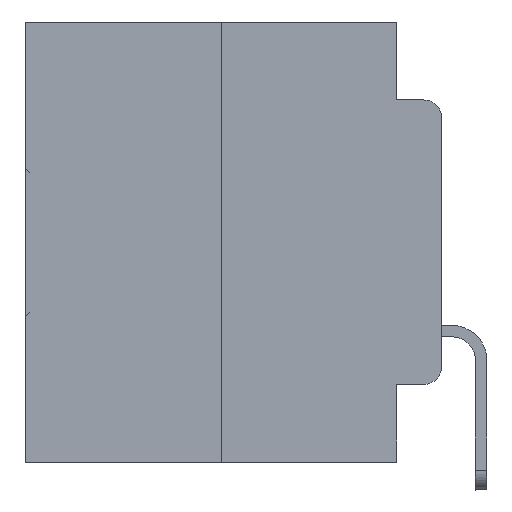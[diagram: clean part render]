
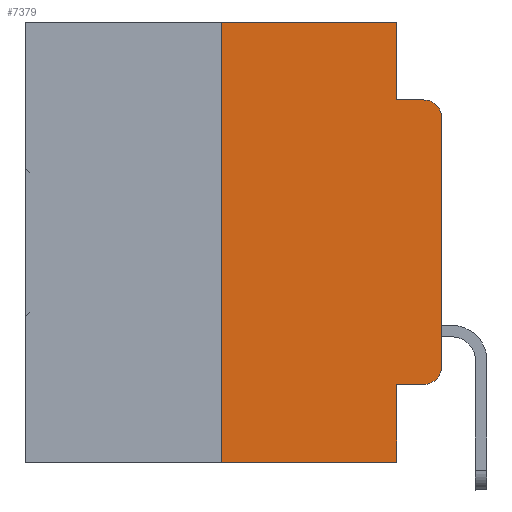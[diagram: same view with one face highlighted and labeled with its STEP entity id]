
A CAD part, left-side view. The second image highlights one B-rep face of the part: STEP entity #7379.
In plain terms, the highlighted planar face has unit normal (-1, 0, 0).
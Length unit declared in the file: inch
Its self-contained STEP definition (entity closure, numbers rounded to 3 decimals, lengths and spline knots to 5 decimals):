
#583 = ORIENTED_EDGE ( 'NONE', *, *, #6155, .T. ) ;
#1033 = DIRECTION ( 'NONE',  ( 0., 0., -1. ) ) ;
#2164 = VERTEX_POINT ( 'NONE', #14094 ) ;
#2459 = CARTESIAN_POINT ( 'NONE',  ( 0., 0.051, -0.4115 ) ) ;
#3384 = CARTESIAN_POINT ( 'NONE',  ( 0., 0.051, 0. ) ) ;
#4004 = ORIENTED_EDGE ( 'NONE', *, *, #21494, .F. ) ;
#4017 = CARTESIAN_POINT ( 'NONE',  ( 0., 0., -0.3915 ) ) ;
#4564 = VERTEX_POINT ( 'NONE', #2459 ) ;
#4943 = VECTOR ( 'NONE', #14178, 39.37008 ) ;
#5143 = LINE ( 'NONE', #29295, #17501 ) ;
#5818 = CARTESIAN_POINT ( 'NONE',  ( 0., 0.02, -0.4115 ) ) ;
#6155 = EDGE_CURVE ( 'NONE', #23217, #22985, #13367, .T. ) ;
#6268 = DIRECTION ( 'NONE',  ( -1., 0., 0. ) ) ;
#6496 = VECTOR ( 'NONE', #7029, 39.37008 ) ;
#6541 = AXIS2_PLACEMENT_3D ( 'NONE', #14910, #22214, #17453 ) ;
#6672 = EDGE_CURVE ( 'NONE', #29291, #15636, #27678, .T. ) ;
#6711 = CARTESIAN_POINT ( 'NONE',  ( 0., 0.02, -0.0885 ) ) ;
#7029 = DIRECTION ( 'NONE',  ( 0., -1., 0. ) ) ;
#7379 = ADVANCED_FACE ( 'NONE', ( #26851 ), #12520, .F. ) ;
#8133 = CARTESIAN_POINT ( 'NONE',  ( 0., 0.25, -0.5 ) ) ;
#8259 = VERTEX_POINT ( 'NONE', #17502 ) ;
#8344 = EDGE_CURVE ( 'NONE', #2164, #8259, #5143, .T. ) ;
#8502 = ORIENTED_EDGE ( 'NONE', *, *, #29408, .T. ) ;
#10114 = DIRECTION ( 'NONE',  ( 0., 0., 1. ) ) ;
#10580 = CARTESIAN_POINT ( 'NONE',  ( 0., 0.25, 0. ) ) ;
#10733 = ORIENTED_EDGE ( 'NONE', *, *, #30667, .F. ) ;
#11761 = CARTESIAN_POINT ( 'NONE',  ( 0., 0.02, -0.1085 ) ) ;
#11800 = DIRECTION ( 'NONE',  ( 0., 0., -1. ) ) ;
#11861 = AXIS2_PLACEMENT_3D ( 'NONE', #11761, #16076, #30893 ) ;
#12502 = VECTOR ( 'NONE', #11800, 39.37008 ) ;
#12520 = PLANE ( 'NONE',  #6541 ) ;
#12724 = DIRECTION ( 'NONE',  ( 0., -1., 0. ) ) ;
#12953 = EDGE_CURVE ( 'NONE', #13323, #2164, #29362, .T. ) ;
#13323 = VERTEX_POINT ( 'NONE', #8133 ) ;
#13367 = CIRCLE ( 'NONE', #11861, 0.02 ) ;
#13442 = EDGE_LOOP ( 'NONE', ( #8502, #583, #24072, #4004, #18825, #17310, #15193, #10733, #26662, #17762 ) ) ;
#14094 = CARTESIAN_POINT ( 'NONE',  ( 0., 0.25, 0. ) ) ;
#14178 = DIRECTION ( 'NONE',  ( 0., 0., 1. ) ) ;
#14910 = CARTESIAN_POINT ( 'NONE',  ( 0., 0.473, 0. ) ) ;
#15193 = ORIENTED_EDGE ( 'NONE', *, *, #31333, .T. ) ;
#15636 = VERTEX_POINT ( 'NONE', #4017 ) ;
#16076 = DIRECTION ( 'NONE',  ( -1., 0., 0. ) ) ;
#16433 = LINE ( 'NONE', #26139, #26020 ) ;
#17168 = LINE ( 'NONE', #26881, #6496 ) ;
#17310 = ORIENTED_EDGE ( 'NONE', *, *, #12953, .F. ) ;
#17453 = DIRECTION ( 'NONE',  ( 0., 0., -1. ) ) ;
#17501 = VECTOR ( 'NONE', #12724, 39.37008 ) ;
#17502 = CARTESIAN_POINT ( 'NONE',  ( 0., 0.051, 0. ) ) ;
#17695 = CARTESIAN_POINT ( 'NONE',  ( 0., 0.051, -0.5 ) ) ;
#17762 = ORIENTED_EDGE ( 'NONE', *, *, #6672, .T. ) ;
#18314 = CARTESIAN_POINT ( 'NONE',  ( 0., 0.02, -0.3915 ) ) ;
#18342 = CARTESIAN_POINT ( 'NONE',  ( 0., 0.051, -0.4115 ) ) ;
#18641 = CARTESIAN_POINT ( 'NONE',  ( 0., 0., 0. ) ) ;
#18825 = ORIENTED_EDGE ( 'NONE', *, *, #8344, .F. ) ;
#20395 = LINE ( 'NONE', #18342, #29828 ) ;
#20563 = DIRECTION ( 'NONE',  ( 0., -1., 0. ) ) ;
#20739 = VECTOR ( 'NONE', #10114, 39.37008 ) ;
#21083 = VERTEX_POINT ( 'NONE', #17695 ) ;
#21494 = EDGE_CURVE ( 'NONE', #8259, #22904, #22576, .T. ) ;
#22214 = DIRECTION ( 'NONE',  ( 1., 0., 0. ) ) ;
#22394 = CARTESIAN_POINT ( 'NONE',  ( 0., 0., -0.1085 ) ) ;
#22576 = LINE ( 'NONE', #3384, #30796 ) ;
#22904 = VERTEX_POINT ( 'NONE', #23383 ) ;
#22985 = VERTEX_POINT ( 'NONE', #6711 ) ;
#23080 = AXIS2_PLACEMENT_3D ( 'NONE', #18314, #6268, #1033 ) ;
#23217 = VERTEX_POINT ( 'NONE', #22394 ) ;
#23383 = CARTESIAN_POINT ( 'NONE',  ( 0., 0.051, -0.0885 ) ) ;
#23589 = CARTESIAN_POINT ( 'NONE',  ( 0., 0.051, 0. ) ) ;
#24072 = ORIENTED_EDGE ( 'NONE', *, *, #25575, .F. ) ;
#25575 = EDGE_CURVE ( 'NONE', #22904, #22985, #16433, .T. ) ;
#25972 = LINE ( 'NONE', #23589, #12502 ) ;
#26020 = VECTOR ( 'NONE', #20563, 39.37008 ) ;
#26139 = CARTESIAN_POINT ( 'NONE',  ( 0., 0.051, -0.0885 ) ) ;
#26573 = LINE ( 'NONE', #18641, #4943 ) ;
#26662 = ORIENTED_EDGE ( 'NONE', *, *, #30482, .T. ) ;
#26851 = FACE_OUTER_BOUND ( 'NONE', #13442, .T. ) ;
#26881 = CARTESIAN_POINT ( 'NONE',  ( 0., 0.473, -0.5 ) ) ;
#27678 = CIRCLE ( 'NONE', #23080, 0.02 ) ;
#29291 = VERTEX_POINT ( 'NONE', #5818 ) ;
#29295 = CARTESIAN_POINT ( 'NONE',  ( 0., 0.473, 0. ) ) ;
#29362 = LINE ( 'NONE', #10580, #20739 ) ;
#29408 = EDGE_CURVE ( 'NONE', #15636, #23217, #26573, .T. ) ;
#29791 = DIRECTION ( 'NONE',  ( 0., 0., -1. ) ) ;
#29828 = VECTOR ( 'NONE', #30311, 39.37008 ) ;
#30311 = DIRECTION ( 'NONE',  ( 0., -1., 0. ) ) ;
#30482 = EDGE_CURVE ( 'NONE', #4564, #29291, #20395, .T. ) ;
#30667 = EDGE_CURVE ( 'NONE', #4564, #21083, #25972, .T. ) ;
#30796 = VECTOR ( 'NONE', #29791, 39.37008 ) ;
#30893 = DIRECTION ( 'NONE',  ( 0., 0., -1. ) ) ;
#31333 = EDGE_CURVE ( 'NONE', #13323, #21083, #17168, .T. ) ;
